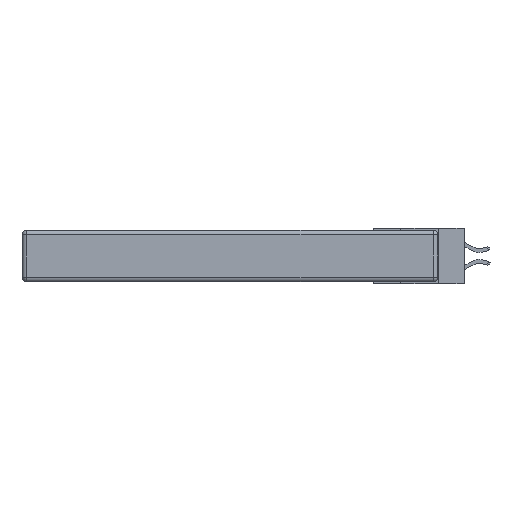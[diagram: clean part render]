
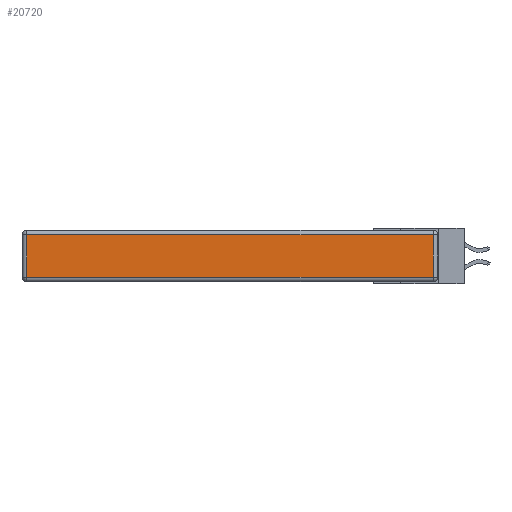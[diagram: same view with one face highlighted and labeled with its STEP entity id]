
A CAD part, left-side view. The second image highlights one B-rep face of the part: STEP entity #20720.
In plain terms, the highlighted planar face has unit normal (-1, 0, 0).
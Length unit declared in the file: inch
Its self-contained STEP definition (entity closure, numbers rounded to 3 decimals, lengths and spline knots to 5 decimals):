
#1773 = ORIENTED_EDGE ( 'NONE', *, *, #22075, .T. ) ;
#2705 = ORIENTED_EDGE ( 'NONE', *, *, #14961, .T. ) ;
#2883 = VECTOR ( 'NONE', #14693, 39.37008 ) ;
#4120 = DIRECTION ( 'NONE',  ( 0., 1., 0. ) ) ;
#4400 = EDGE_CURVE ( 'NONE', #24496, #28432, #9458, .T. ) ;
#4422 = CARTESIAN_POINT ( 'NONE',  ( 0., 0.03, -0.03 ) ) ;
#6579 = PLANE ( 'NONE',  #19860 ) ;
#7282 = FACE_OUTER_BOUND ( 'NONE', #15400, .T. ) ;
#7315 = LINE ( 'NONE', #7545, #23813 ) ;
#7545 = CARTESIAN_POINT ( 'NONE',  ( 0., 0.03, -0.343 ) ) ;
#7612 = ORIENTED_EDGE ( 'NONE', *, *, #4400, .T. ) ;
#9458 = LINE ( 'NONE', #28431, #2883 ) ;
#11026 = CARTESIAN_POINT ( 'NONE',  ( 0., 2.75, -0.03 ) ) ;
#12117 = LINE ( 'NONE', #26994, #29726 ) ;
#12988 = DIRECTION ( 'NONE',  ( 0., 0., -1. ) ) ;
#14059 = LINE ( 'NONE', #11026, #22268 ) ;
#14236 = CARTESIAN_POINT ( 'NONE',  ( 0., 0.03, -0.313 ) ) ;
#14693 = DIRECTION ( 'NONE',  ( 0., -1., 0. ) ) ;
#14961 = EDGE_CURVE ( 'NONE', #28432, #20841, #7315, .T. ) ;
#15400 = EDGE_LOOP ( 'NONE', ( #7612, #2705, #1773, #26884 ) ) ;
#17861 = DIRECTION ( 'NONE',  ( 0., 0., 1. ) ) ;
#18155 = CARTESIAN_POINT ( 'NONE',  ( 0., 0., -0.343 ) ) ;
#18818 = CARTESIAN_POINT ( 'NONE',  ( 0., 2.72, -0.313 ) ) ;
#19860 = AXIS2_PLACEMENT_3D ( 'NONE', #18155, #26972, #17861 ) ;
#19996 = DIRECTION ( 'NONE',  ( 0., 0., 1. ) ) ;
#20720 = ADVANCED_FACE ( 'NONE', ( #7282 ), #6579, .T. ) ;
#20841 = VERTEX_POINT ( 'NONE', #4422 ) ;
#22075 = EDGE_CURVE ( 'NONE', #20841, #23706, #14059, .T. ) ;
#22268 = VECTOR ( 'NONE', #4120, 39.37008 ) ;
#23352 = CARTESIAN_POINT ( 'NONE',  ( 0., 2.72, -0.03 ) ) ;
#23706 = VERTEX_POINT ( 'NONE', #23352 ) ;
#23813 = VECTOR ( 'NONE', #19996, 39.37008 ) ;
#24496 = VERTEX_POINT ( 'NONE', #18818 ) ;
#26884 = ORIENTED_EDGE ( 'NONE', *, *, #28214, .T. ) ;
#26972 = DIRECTION ( 'NONE',  ( -1., 0., 0. ) ) ;
#26994 = CARTESIAN_POINT ( 'NONE',  ( 0., 2.72, -0.343 ) ) ;
#28214 = EDGE_CURVE ( 'NONE', #23706, #24496, #12117, .T. ) ;
#28431 = CARTESIAN_POINT ( 'NONE',  ( 0., 0., -0.313 ) ) ;
#28432 = VERTEX_POINT ( 'NONE', #14236 ) ;
#29726 = VECTOR ( 'NONE', #12988, 39.37008 ) ;
